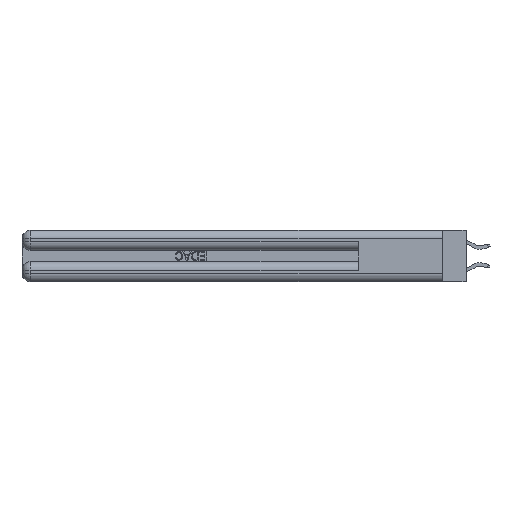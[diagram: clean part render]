
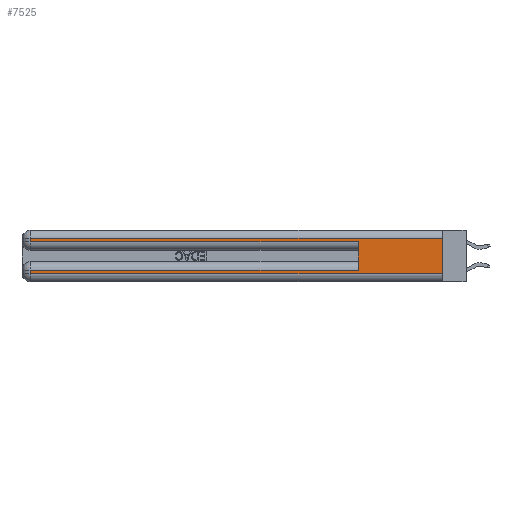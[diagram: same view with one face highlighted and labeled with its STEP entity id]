
A CAD part, left-side view. The second image highlights one B-rep face of the part: STEP entity #7525.
In plain terms, the highlighted planar face has unit normal (-1, 0, 0).
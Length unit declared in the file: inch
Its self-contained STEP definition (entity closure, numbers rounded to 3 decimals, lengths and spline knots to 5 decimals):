
#94 = VECTOR ( 'NONE', #12264, 39.37008 ) ;
#161 = LINE ( 'NONE', #21044, #22378 ) ;
#847 = ORIENTED_EDGE ( 'NONE', *, *, #11752, .T. ) ;
#1062 = CARTESIAN_POINT ( 'NONE',  ( 0., 0.6, 0.285 ) ) ;
#1137 = CARTESIAN_POINT ( 'NONE',  ( 0., 2.94, 0.31 ) ) ;
#1412 = CARTESIAN_POINT ( 'NONE',  ( 0., 2.94, 0.285 ) ) ;
#2210 = ORIENTED_EDGE ( 'NONE', *, *, #12792, .T. ) ;
#2685 = EDGE_CURVE ( 'NONE', #20820, #15547, #4715, .T. ) ;
#3084 = DIRECTION ( 'NONE',  ( 0., 0., -1. ) ) ;
#3669 = EDGE_CURVE ( 'NONE', #5374, #26707, #27420, .T. ) ;
#4715 = LINE ( 'NONE', #26596, #26804 ) ;
#5094 = VERTEX_POINT ( 'NONE', #1062 ) ;
#5374 = VERTEX_POINT ( 'NONE', #17049 ) ;
#5819 = CARTESIAN_POINT ( 'NONE',  ( 0., 0., 0.31 ) ) ;
#5853 = CARTESIAN_POINT ( 'NONE',  ( 0., 2.94, 0.37 ) ) ;
#6674 = EDGE_CURVE ( 'NONE', #14418, #24056, #22575, .T. ) ;
#6771 = DIRECTION ( 'NONE',  ( 0., 0., -1. ) ) ;
#7220 = EDGE_LOOP ( 'NONE', ( #27334, #10992, #22370, #847, #18761, #24370, #2210, #8629 ) ) ;
#7525 = ADVANCED_FACE ( 'NONE', ( #21561 ), #7856, .F. ) ;
#7856 = PLANE ( 'NONE',  #26949 ) ;
#8416 = DIRECTION ( 'NONE',  ( 0., 1., 0. ) ) ;
#8629 = ORIENTED_EDGE ( 'NONE', *, *, #6674, .T. ) ;
#10260 = LINE ( 'NONE', #5853, #94 ) ;
#10593 = LINE ( 'NONE', #17540, #15688 ) ;
#10992 = ORIENTED_EDGE ( 'NONE', *, *, #13437, .T. ) ;
#11638 = VECTOR ( 'NONE', #24089, 39.37008 ) ;
#11752 = EDGE_CURVE ( 'NONE', #15547, #5094, #23014, .T. ) ;
#12201 = DIRECTION ( 'NONE',  ( 0., 0., -1. ) ) ;
#12264 = DIRECTION ( 'NONE',  ( 0., 0., -1. ) ) ;
#12525 = DIRECTION ( 'NONE',  ( 0., 0., 1. ) ) ;
#12792 = EDGE_CURVE ( 'NONE', #26707, #14418, #10260, .T. ) ;
#13437 = EDGE_CURVE ( 'NONE', #25347, #20820, #18325, .T. ) ;
#14418 = VERTEX_POINT ( 'NONE', #26961 ) ;
#15547 = VERTEX_POINT ( 'NONE', #1412 ) ;
#15688 = VECTOR ( 'NONE', #6771, 39.37008 ) ;
#16165 = VECTOR ( 'NONE', #8416, 39.37008 ) ;
#16281 = CARTESIAN_POINT ( 'NONE',  ( 0., 0., 0.31 ) ) ;
#16680 = CARTESIAN_POINT ( 'NONE',  ( 0., 2.94, 0.085 ) ) ;
#16955 = VECTOR ( 'NONE', #24461, 39.37008 ) ;
#17049 = CARTESIAN_POINT ( 'NONE',  ( 0., 0.6, 0.085 ) ) ;
#17540 = CARTESIAN_POINT ( 'NONE',  ( 0., 0., 0.37 ) ) ;
#17702 = CARTESIAN_POINT ( 'NONE',  ( 0., 0., 0.285 ) ) ;
#18325 = LINE ( 'NONE', #5819, #23277 ) ;
#18566 = EDGE_CURVE ( 'NONE', #5374, #5094, #161, .T. ) ;
#18761 = ORIENTED_EDGE ( 'NONE', *, *, #18566, .F. ) ;
#20390 = CARTESIAN_POINT ( 'NONE',  ( 0., 0., 0.06 ) ) ;
#20820 = VERTEX_POINT ( 'NONE', #1137 ) ;
#21044 = CARTESIAN_POINT ( 'NONE',  ( 0., 0.6, 0.145 ) ) ;
#21288 = CARTESIAN_POINT ( 'NONE',  ( 0., 0., 0.085 ) ) ;
#21561 = FACE_OUTER_BOUND ( 'NONE', #7220, .T. ) ;
#22330 = CARTESIAN_POINT ( 'NONE',  ( 0., 0., 0.06 ) ) ;
#22370 = ORIENTED_EDGE ( 'NONE', *, *, #2685, .T. ) ;
#22378 = VECTOR ( 'NONE', #12525, 39.37008 ) ;
#22575 = LINE ( 'NONE', #22330, #16955 ) ;
#22850 = CARTESIAN_POINT ( 'NONE',  ( 0., 0., 0.37 ) ) ;
#23014 = LINE ( 'NONE', #17702, #11638 ) ;
#23277 = VECTOR ( 'NONE', #25092, 39.37008 ) ;
#24056 = VERTEX_POINT ( 'NONE', #20390 ) ;
#24089 = DIRECTION ( 'NONE',  ( 0., -1., 0. ) ) ;
#24370 = ORIENTED_EDGE ( 'NONE', *, *, #3669, .T. ) ;
#24461 = DIRECTION ( 'NONE',  ( 0., -1., 0. ) ) ;
#24972 = DIRECTION ( 'NONE',  ( 1., 0., 0. ) ) ;
#25092 = DIRECTION ( 'NONE',  ( 0., 1., 0. ) ) ;
#25347 = VERTEX_POINT ( 'NONE', #16281 ) ;
#26368 = EDGE_CURVE ( 'NONE', #25347, #24056, #10593, .T. ) ;
#26596 = CARTESIAN_POINT ( 'NONE',  ( 0., 2.94, 0.37 ) ) ;
#26707 = VERTEX_POINT ( 'NONE', #16680 ) ;
#26804 = VECTOR ( 'NONE', #3084, 39.37008 ) ;
#26949 = AXIS2_PLACEMENT_3D ( 'NONE', #22850, #24972, #12201 ) ;
#26961 = CARTESIAN_POINT ( 'NONE',  ( 0., 2.94, 0.06 ) ) ;
#27334 = ORIENTED_EDGE ( 'NONE', *, *, #26368, .F. ) ;
#27420 = LINE ( 'NONE', #21288, #16165 ) ;
